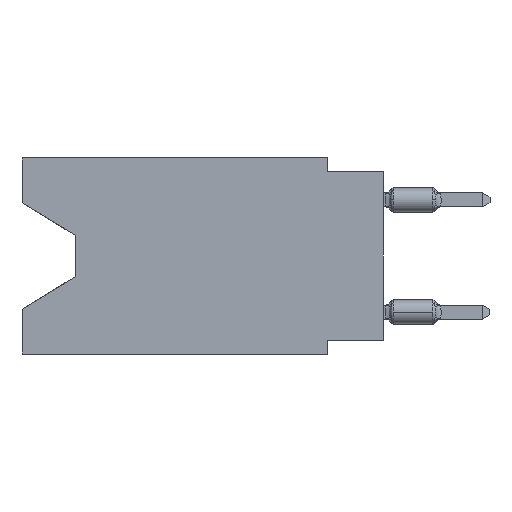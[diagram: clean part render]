
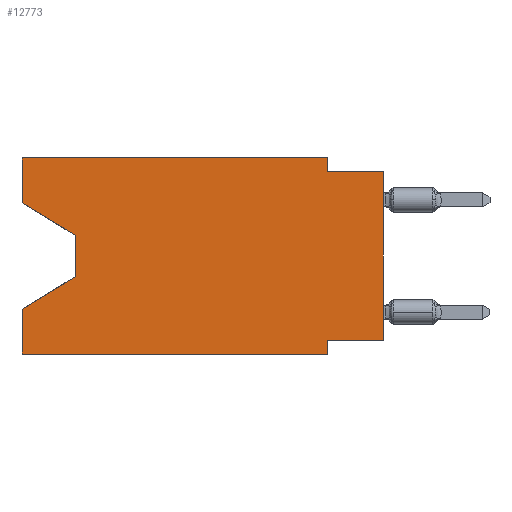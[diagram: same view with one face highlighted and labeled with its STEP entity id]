
A CAD part, left-side view. The second image highlights one B-rep face of the part: STEP entity #12773.
In plain terms, the highlighted planar face has unit normal (-1, 0, 0).
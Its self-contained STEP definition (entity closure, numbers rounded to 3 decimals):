
#105 = CARTESIAN_POINT ( 'NONE',  ( 0., 2.54, -8.89 ) ) ;
#394 = DIRECTION ( 'NONE',  ( 0., 0., -1. ) ) ;
#480 = VERTEX_POINT ( 'NONE', #7208 ) ;
#494 = ORIENTED_EDGE ( 'NONE', *, *, #6113, .T. ) ;
#534 = VERTEX_POINT ( 'NONE', #9069 ) ;
#1288 = DIRECTION ( 'NONE',  ( 0., 0., -1. ) ) ;
#1315 = LINE ( 'NONE', #11164, #6761 ) ;
#1334 = CARTESIAN_POINT ( 'NONE',  ( 0., 16.383, 0. ) ) ;
#1594 = VERTEX_POINT ( 'NONE', #8513 ) ;
#2212 = CARTESIAN_POINT ( 'NONE',  ( 0., 16.383, -6.852 ) ) ;
#2764 = VERTEX_POINT ( 'NONE', #19958 ) ;
#3079 = DIRECTION ( 'NONE',  ( 0., 0., -1. ) ) ;
#3859 = CARTESIAN_POINT ( 'NONE',  ( 0., 0., -8.255 ) ) ;
#3906 = DIRECTION ( 'NONE',  ( 0., 0.855, -0.519 ) ) ;
#4068 = DIRECTION ( 'NONE',  ( 0., 1., 0. ) ) ;
#4186 = CARTESIAN_POINT ( 'NONE',  ( 0., 0., -0.635 ) ) ;
#4207 = EDGE_CURVE ( 'NONE', #17226, #1594, #9378, .T. ) ;
#4220 = LINE ( 'NONE', #20446, #9901 ) ;
#4484 = ORIENTED_EDGE ( 'NONE', *, *, #6518, .F. ) ;
#4606 = LINE ( 'NONE', #6019, #10978 ) ;
#5093 = DIRECTION ( 'NONE',  ( 0., -0.855, -0.519 ) ) ;
#5116 = VERTEX_POINT ( 'NONE', #10194 ) ;
#5152 = EDGE_CURVE ( 'NONE', #480, #1594, #15736, .T. ) ;
#5386 = VERTEX_POINT ( 'NONE', #17811 ) ;
#5541 = DIRECTION ( 'NONE',  ( 1., 0., 0. ) ) ;
#5616 = DIRECTION ( 'NONE',  ( 0., -1., 0. ) ) ;
#6019 = CARTESIAN_POINT ( 'NONE',  ( 0., 16.383, 0. ) ) ;
#6037 = CARTESIAN_POINT ( 'NONE',  ( 0., 0., -8.255 ) ) ;
#6113 = EDGE_CURVE ( 'NONE', #5386, #16108, #4220, .T. ) ;
#6249 = ORIENTED_EDGE ( 'NONE', *, *, #12086, .T. ) ;
#6474 = DIRECTION ( 'NONE',  ( 0., 0., 1. ) ) ;
#6518 = EDGE_CURVE ( 'NONE', #7301, #15254, #20538, .T. ) ;
#6761 = VECTOR ( 'NONE', #3079, 1000. ) ;
#7208 = CARTESIAN_POINT ( 'NONE',  ( 0., 2.54, -0.635 ) ) ;
#7301 = VERTEX_POINT ( 'NONE', #12212 ) ;
#7452 = LINE ( 'NONE', #18295, #17434 ) ;
#7569 = ORIENTED_EDGE ( 'NONE', *, *, #4207, .T. ) ;
#7746 = ORIENTED_EDGE ( 'NONE', *, *, #20006, .F. ) ;
#8513 = CARTESIAN_POINT ( 'NONE',  ( 0., 0., -0.635 ) ) ;
#8530 = VECTOR ( 'NONE', #5616, 1000. ) ;
#8531 = EDGE_CURVE ( 'NONE', #17817, #2764, #7452, .T. ) ;
#8608 = ORIENTED_EDGE ( 'NONE', *, *, #16923, .T. ) ;
#8669 = CARTESIAN_POINT ( 'NONE',  ( 0., 2.54, -8.255 ) ) ;
#9069 = CARTESIAN_POINT ( 'NONE',  ( 0., 16.383, -8.89 ) ) ;
#9128 = ORIENTED_EDGE ( 'NONE', *, *, #11844, .F. ) ;
#9378 = LINE ( 'NONE', #19624, #11414 ) ;
#9803 = DIRECTION ( 'NONE',  ( 0., 0., 1. ) ) ;
#9901 = VECTOR ( 'NONE', #3906, 1000. ) ;
#10194 = CARTESIAN_POINT ( 'NONE',  ( 0., 2.54, -8.89 ) ) ;
#10565 = FACE_OUTER_BOUND ( 'NONE', #20790, .T. ) ;
#10978 = VECTOR ( 'NONE', #19326, 1000. ) ;
#11164 = CARTESIAN_POINT ( 'NONE',  ( 0., 2.54, 0. ) ) ;
#11414 = VECTOR ( 'NONE', #9803, 1000. ) ;
#11727 = DIRECTION ( 'NONE',  ( 0., -1., 0. ) ) ;
#11844 = EDGE_CURVE ( 'NONE', #15254, #480, #1315, .T. ) ;
#12086 = EDGE_CURVE ( 'NONE', #2764, #5386, #16242, .T. ) ;
#12212 = CARTESIAN_POINT ( 'NONE',  ( 0., 16.383, 0. ) ) ;
#12561 = VECTOR ( 'NONE', #4068, 1000. ) ;
#12773 = ADVANCED_FACE ( 'NONE', ( #10565 ), #17208, .F. ) ;
#12951 = VECTOR ( 'NONE', #11727, 1000. ) ;
#13281 = ORIENTED_EDGE ( 'NONE', *, *, #5152, .F. ) ;
#13412 = DIRECTION ( 'NONE',  ( 0., 0., -1. ) ) ;
#13762 = LINE ( 'NONE', #3859, #12561 ) ;
#14063 = CARTESIAN_POINT ( 'NONE',  ( 0., 2.54, 0. ) ) ;
#14244 = VECTOR ( 'NONE', #19118, 1000. ) ;
#14768 = CARTESIAN_POINT ( 'NONE',  ( 0., 16.383, -8.89 ) ) ;
#14919 = CARTESIAN_POINT ( 'NONE',  ( 0., 13.97, -3.505 ) ) ;
#14975 = AXIS2_PLACEMENT_3D ( 'NONE', #15348, #5541, #394 ) ;
#15054 = LINE ( 'NONE', #105, #17911 ) ;
#15204 = LINE ( 'NONE', #14768, #12951 ) ;
#15254 = VERTEX_POINT ( 'NONE', #14063 ) ;
#15348 = CARTESIAN_POINT ( 'NONE',  ( 0., 16.383, 0. ) ) ;
#15736 = LINE ( 'NONE', #4186, #14244 ) ;
#15914 = EDGE_CURVE ( 'NONE', #534, #16108, #17939, .T. ) ;
#16108 = VERTEX_POINT ( 'NONE', #2212 ) ;
#16157 = VECTOR ( 'NONE', #1288, 1000. ) ;
#16242 = LINE ( 'NONE', #14919, #16157 ) ;
#16298 = ORIENTED_EDGE ( 'NONE', *, *, #19064, .F. ) ;
#16923 = EDGE_CURVE ( 'NONE', #534, #5116, #15204, .T. ) ;
#17174 = CARTESIAN_POINT ( 'NONE',  ( 0., 16.383, 0. ) ) ;
#17208 = PLANE ( 'NONE',  #14975 ) ;
#17226 = VERTEX_POINT ( 'NONE', #6037 ) ;
#17434 = VECTOR ( 'NONE', #5093, 1000. ) ;
#17811 = CARTESIAN_POINT ( 'NONE',  ( 0., 13.97, -5.385 ) ) ;
#17817 = VERTEX_POINT ( 'NONE', #20572 ) ;
#17911 = VECTOR ( 'NONE', #13412, 1000. ) ;
#17939 = LINE ( 'NONE', #1334, #18505 ) ;
#18120 = VERTEX_POINT ( 'NONE', #8669 ) ;
#18295 = CARTESIAN_POINT ( 'NONE',  ( 0., 16.383, -2.038 ) ) ;
#18505 = VECTOR ( 'NONE', #6474, 1000. ) ;
#18696 = ORIENTED_EDGE ( 'NONE', *, *, #15914, .F. ) ;
#18796 = EDGE_CURVE ( 'NONE', #17226, #18120, #13762, .T. ) ;
#18837 = ORIENTED_EDGE ( 'NONE', *, *, #8531, .T. ) ;
#19064 = EDGE_CURVE ( 'NONE', #18120, #5116, #15054, .T. ) ;
#19118 = DIRECTION ( 'NONE',  ( 0., -1., 0. ) ) ;
#19326 = DIRECTION ( 'NONE',  ( 0., 0., 1. ) ) ;
#19624 = CARTESIAN_POINT ( 'NONE',  ( 0., 0., 0. ) ) ;
#19958 = CARTESIAN_POINT ( 'NONE',  ( 0., 13.97, -3.505 ) ) ;
#20006 = EDGE_CURVE ( 'NONE', #17817, #7301, #4606, .T. ) ;
#20446 = CARTESIAN_POINT ( 'NONE',  ( 0., 13.97, -5.385 ) ) ;
#20538 = LINE ( 'NONE', #17174, #8530 ) ;
#20572 = CARTESIAN_POINT ( 'NONE',  ( 0., 16.383, -2.038 ) ) ;
#20790 = EDGE_LOOP ( 'NONE', ( #18837, #6249, #494, #18696, #8608, #16298, #20848, #7569, #13281, #9128, #4484, #7746 ) ) ;
#20848 = ORIENTED_EDGE ( 'NONE', *, *, #18796, .F. ) ;
